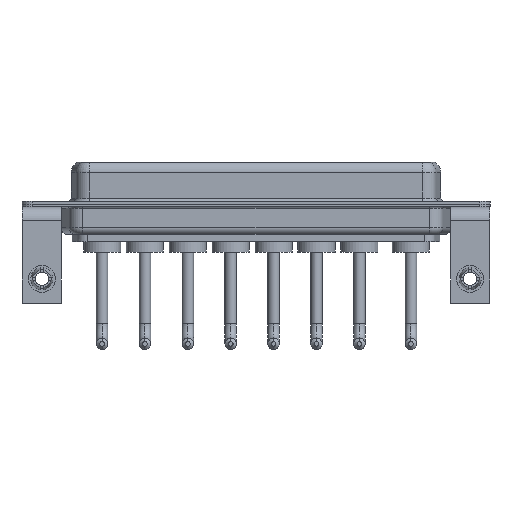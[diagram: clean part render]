
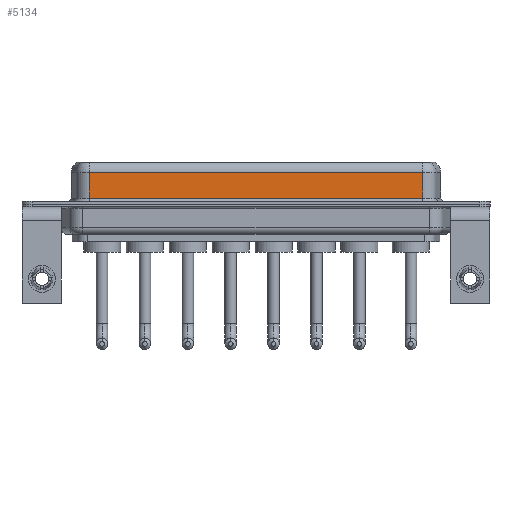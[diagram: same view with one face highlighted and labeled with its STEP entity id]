
A CAD part, front view. The second image highlights one B-rep face of the part: STEP entity #5134.
In plain terms, the highlighted planar face has unit normal (0, -1, 0).
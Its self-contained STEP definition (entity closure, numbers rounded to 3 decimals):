
#117 = VECTOR ( 'NONE', #6897, 1000. ) ;
#1311 = DIRECTION ( 'NONE',  ( -1., 0., 0. ) ) ;
#1520 = CARTESIAN_POINT ( 'NONE',  ( 56.462, -3.95, 0.9 ) ) ;
#1970 = DIRECTION ( 'NONE',  ( 0., 1., 0. ) ) ;
#2785 = VECTOR ( 'NONE', #1311, 1000. ) ;
#2907 = CARTESIAN_POINT ( 'NONE',  ( 7.038, -3.95, 4.65 ) ) ;
#3158 = EDGE_CURVE ( 'NONE', #6887, #9680, #12241, .T. ) ;
#3301 = ORIENTED_EDGE ( 'NONE', *, *, #6194, .F. ) ;
#4137 = VECTOR ( 'NONE', #10493, 1000. ) ;
#4355 = FACE_OUTER_BOUND ( 'NONE', #4524, .T. ) ;
#4483 = VECTOR ( 'NONE', #9679, 1000. ) ;
#4488 = EDGE_CURVE ( 'NONE', #12334, #6887, #5988, .T. ) ;
#4524 = EDGE_LOOP ( 'NONE', ( #3301, #8100, #15467, #6958 ) ) ;
#4550 = LINE ( 'NONE', #15567, #4137 ) ;
#5134 = ADVANCED_FACE ( 'NONE', ( #4355 ), #8073, .F. ) ;
#5196 = CARTESIAN_POINT ( 'NONE',  ( 7.038, -3.95, 6.4 ) ) ;
#5988 = LINE ( 'NONE', #8442, #2785 ) ;
#6133 = AXIS2_PLACEMENT_3D ( 'NONE', #6728, #1970, #6499 ) ;
#6194 = EDGE_CURVE ( 'NONE', #12334, #7750, #4550, .T. ) ;
#6499 = DIRECTION ( 'NONE',  ( 0., 0., 1. ) ) ;
#6728 = CARTESIAN_POINT ( 'NONE',  ( 56.462, -3.95, 6.4 ) ) ;
#6887 = VERTEX_POINT ( 'NONE', #2907 ) ;
#6897 = DIRECTION ( 'NONE',  ( 0., 0., -1. ) ) ;
#6958 = ORIENTED_EDGE ( 'NONE', *, *, #9817, .T. ) ;
#7750 = VERTEX_POINT ( 'NONE', #8977 ) ;
#8073 = PLANE ( 'NONE',  #6133 ) ;
#8100 = ORIENTED_EDGE ( 'NONE', *, *, #4488, .T. ) ;
#8442 = CARTESIAN_POINT ( 'NONE',  ( 56.462, -3.95, 4.65 ) ) ;
#8562 = CARTESIAN_POINT ( 'NONE',  ( 56.462, -3.95, 4.65 ) ) ;
#8570 = LINE ( 'NONE', #1520, #4483 ) ;
#8977 = CARTESIAN_POINT ( 'NONE',  ( 56.462, -3.95, 0.9 ) ) ;
#9679 = DIRECTION ( 'NONE',  ( 1., 0., 0. ) ) ;
#9680 = VERTEX_POINT ( 'NONE', #11832 ) ;
#9817 = EDGE_CURVE ( 'NONE', #9680, #7750, #8570, .T. ) ;
#10493 = DIRECTION ( 'NONE',  ( 0., 0., -1. ) ) ;
#11832 = CARTESIAN_POINT ( 'NONE',  ( 7.038, -3.95, 0.9 ) ) ;
#12241 = LINE ( 'NONE', #5196, #117 ) ;
#12334 = VERTEX_POINT ( 'NONE', #8562 ) ;
#15467 = ORIENTED_EDGE ( 'NONE', *, *, #3158, .T. ) ;
#15567 = CARTESIAN_POINT ( 'NONE',  ( 56.462, -3.95, 6.4 ) ) ;
